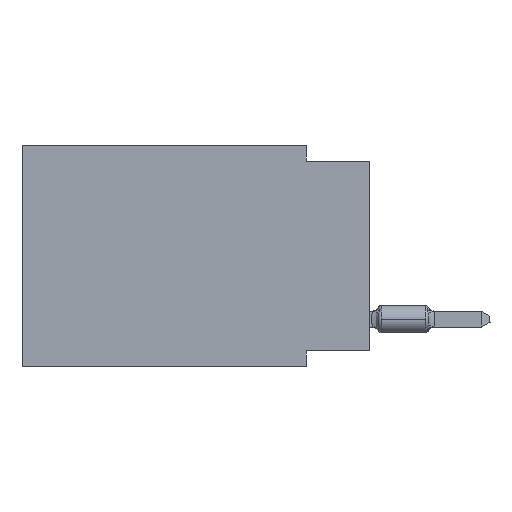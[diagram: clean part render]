
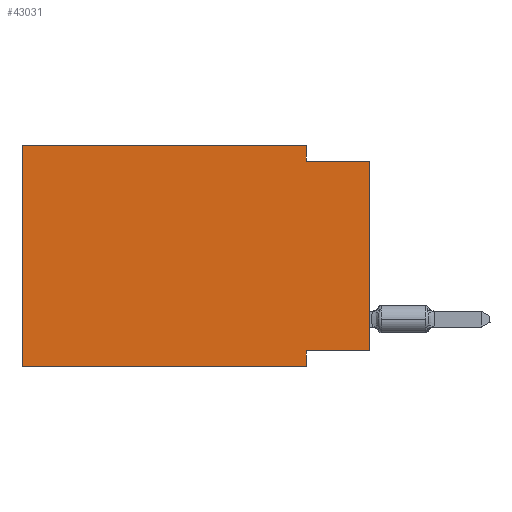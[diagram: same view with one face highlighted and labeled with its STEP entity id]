
A CAD part, left-side view. The second image highlights one B-rep face of the part: STEP entity #43031.
In plain terms, the highlighted planar face has unit normal (-1, 0, 0).
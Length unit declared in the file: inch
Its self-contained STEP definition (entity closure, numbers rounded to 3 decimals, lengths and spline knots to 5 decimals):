
#843 = ORIENTED_EDGE ( 'NONE', *, *, #25140, .T. ) ;
#5279 = DIRECTION ( 'NONE',  ( 0., -1., 0. ) ) ;
#6162 = AXIS2_PLACEMENT_3D ( 'NONE', #17490, #113827, #79578 ) ;
#6496 = LINE ( 'NONE', #41904, #104101 ) ;
#8200 = VECTOR ( 'NONE', #29334, 39.37008 ) ;
#8813 = PLANE ( 'NONE',  #6162 ) ;
#9009 = VECTOR ( 'NONE', #79955, 39.37008 ) ;
#11926 = EDGE_CURVE ( 'NONE', #24500, #100322, #6496, .T. ) ;
#12367 = ORIENTED_EDGE ( 'NONE', *, *, #95751, .F. ) ;
#14173 = ORIENTED_EDGE ( 'NONE', *, *, #11926, .F. ) ;
#14468 = LINE ( 'NONE', #34130, #24876 ) ;
#16109 = DIRECTION ( 'NONE',  ( 0., 0., 1. ) ) ;
#16662 = CARTESIAN_POINT ( 'NONE',  ( 0., 0.55, 0. ) ) ;
#17490 = CARTESIAN_POINT ( 'NONE',  ( 0., 0.55, 0. ) ) ;
#17882 = LINE ( 'NONE', #34728, #53447 ) ;
#19446 = CARTESIAN_POINT ( 'NONE',  ( 0., 0., -0.325 ) ) ;
#22109 = LINE ( 'NONE', #95180, #97651 ) ;
#22175 = CARTESIAN_POINT ( 'NONE',  ( 0., 0.1, -0.025 ) ) ;
#22343 = CARTESIAN_POINT ( 'NONE',  ( 0., 0.1, -0.35 ) ) ;
#23977 = EDGE_CURVE ( 'NONE', #92985, #24500, #50921, .T. ) ;
#24500 = VERTEX_POINT ( 'NONE', #79195 ) ;
#24876 = VECTOR ( 'NONE', #114231, 39.37008 ) ;
#25140 = EDGE_CURVE ( 'NONE', #92985, #58986, #22109, .T. ) ;
#27287 = DIRECTION ( 'NONE',  ( 0., -1., 0. ) ) ;
#29334 = DIRECTION ( 'NONE',  ( 0., 0., -1. ) ) ;
#29486 = ORIENTED_EDGE ( 'NONE', *, *, #23977, .F. ) ;
#34130 = CARTESIAN_POINT ( 'NONE',  ( 0., 0., 0. ) ) ;
#34728 = CARTESIAN_POINT ( 'NONE',  ( 0., 0.1, 0. ) ) ;
#35075 = VERTEX_POINT ( 'NONE', #58185 ) ;
#35992 = CARTESIAN_POINT ( 'NONE',  ( 0., 0., -0.025 ) ) ;
#37432 = ORIENTED_EDGE ( 'NONE', *, *, #62388, .F. ) ;
#38216 = CARTESIAN_POINT ( 'NONE',  ( 0., 0.1, -0.35 ) ) ;
#38270 = VERTEX_POINT ( 'NONE', #92931 ) ;
#39745 = VECTOR ( 'NONE', #27287, 39.37008 ) ;
#41904 = CARTESIAN_POINT ( 'NONE',  ( 0., 0.55, 0. ) ) ;
#43031 = ADVANCED_FACE ( 'NONE', ( #88303 ), #8813, .F. ) ;
#44566 = LINE ( 'NONE', #96806, #9009 ) ;
#50446 = VERTEX_POINT ( 'NONE', #22175 ) ;
#50921 = LINE ( 'NONE', #16662, #99495 ) ;
#52780 = CARTESIAN_POINT ( 'NONE',  ( 0., 0.55, -0.35 ) ) ;
#52814 = LINE ( 'NONE', #35992, #39745 ) ;
#53447 = VECTOR ( 'NONE', #81110, 39.37008 ) ;
#55350 = ORIENTED_EDGE ( 'NONE', *, *, #62503, .F. ) ;
#58185 = CARTESIAN_POINT ( 'NONE',  ( 0., 0.1, -0.325 ) ) ;
#58986 = VERTEX_POINT ( 'NONE', #38216 ) ;
#62388 = EDGE_CURVE ( 'NONE', #107066, #35075, #44566, .T. ) ;
#62503 = EDGE_CURVE ( 'NONE', #100322, #50446, #17882, .T. ) ;
#66324 = EDGE_LOOP ( 'NONE', ( #77973, #12367, #55350, #14173, #29486, #843, #94530, #37432 ) ) ;
#66447 = LINE ( 'NONE', #22343, #8200 ) ;
#76382 = CARTESIAN_POINT ( 'NONE',  ( 0., 0.1, 0. ) ) ;
#77973 = ORIENTED_EDGE ( 'NONE', *, *, #113599, .T. ) ;
#79195 = CARTESIAN_POINT ( 'NONE',  ( 0., 0.55, 0. ) ) ;
#79578 = DIRECTION ( 'NONE',  ( 0., 0., -1. ) ) ;
#79955 = DIRECTION ( 'NONE',  ( 0., 1., 0. ) ) ;
#81110 = DIRECTION ( 'NONE',  ( 0., 0., -1. ) ) ;
#84198 = EDGE_CURVE ( 'NONE', #35075, #58986, #66447, .T. ) ;
#88303 = FACE_OUTER_BOUND ( 'NONE', #66324, .T. ) ;
#92931 = CARTESIAN_POINT ( 'NONE',  ( 0., 0., -0.025 ) ) ;
#92985 = VERTEX_POINT ( 'NONE', #52780 ) ;
#94530 = ORIENTED_EDGE ( 'NONE', *, *, #84198, .F. ) ;
#95180 = CARTESIAN_POINT ( 'NONE',  ( 0., 0.55, -0.35 ) ) ;
#95267 = DIRECTION ( 'NONE',  ( 0., -1., 0. ) ) ;
#95751 = EDGE_CURVE ( 'NONE', #50446, #38270, #52814, .T. ) ;
#96806 = CARTESIAN_POINT ( 'NONE',  ( 0., 0., -0.325 ) ) ;
#97651 = VECTOR ( 'NONE', #5279, 39.37008 ) ;
#99495 = VECTOR ( 'NONE', #16109, 39.37008 ) ;
#100322 = VERTEX_POINT ( 'NONE', #76382 ) ;
#104101 = VECTOR ( 'NONE', #95267, 39.37008 ) ;
#107066 = VERTEX_POINT ( 'NONE', #19446 ) ;
#113599 = EDGE_CURVE ( 'NONE', #107066, #38270, #14468, .T. ) ;
#113827 = DIRECTION ( 'NONE',  ( 1., 0., 0. ) ) ;
#114231 = DIRECTION ( 'NONE',  ( 0., 0., 1. ) ) ;
